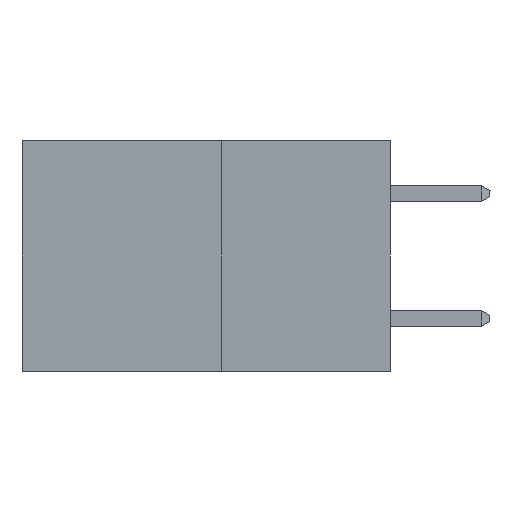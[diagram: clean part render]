
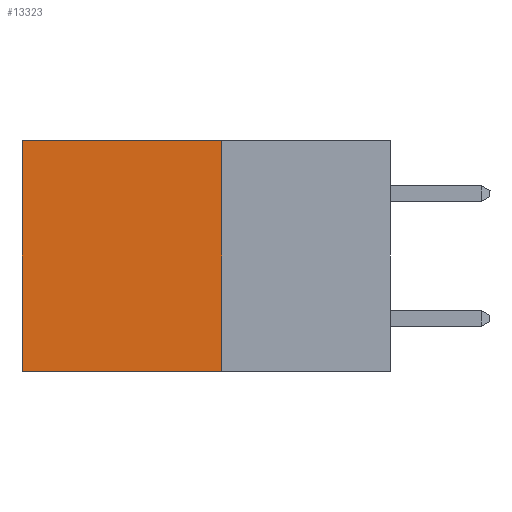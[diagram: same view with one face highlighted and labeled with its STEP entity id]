
A CAD part, left-side view. The second image highlights one B-rep face of the part: STEP entity #13323.
In plain terms, the highlighted planar face has unit normal (-1, 0, 0).
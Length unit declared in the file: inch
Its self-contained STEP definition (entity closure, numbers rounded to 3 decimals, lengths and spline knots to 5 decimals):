
#294 = VECTOR ( 'NONE', #1244, 39.37008 ) ;
#328 = ORIENTED_EDGE ( 'NONE', *, *, #16324, .T. ) ;
#401 = VERTEX_POINT ( 'NONE', #8335 ) ;
#931 = CARTESIAN_POINT ( 'NONE',  ( 0.277, 0.27, -0.37 ) ) ;
#1244 = DIRECTION ( 'NONE',  ( 0., 1., 0. ) ) ;
#3083 = EDGE_CURVE ( 'NONE', #11301, #17555, #4697, .T. ) ;
#3239 = LINE ( 'NONE', #8570, #17644 ) ;
#4622 = AXIS2_PLACEMENT_3D ( 'NONE', #8255, #7303, #7151 ) ;
#4697 = LINE ( 'NONE', #17590, #294 ) ;
#5275 = CARTESIAN_POINT ( 'NONE',  ( 0.277, 0.27, -0.37 ) ) ;
#5292 = DIRECTION ( 'NONE',  ( 0., 0., -1. ) ) ;
#5429 = VECTOR ( 'NONE', #5292, 39.37008 ) ;
#7151 = DIRECTION ( 'NONE',  ( 0., 0., -1. ) ) ;
#7303 = DIRECTION ( 'NONE',  ( 1., 0., 0. ) ) ;
#8029 = CARTESIAN_POINT ( 'NONE',  ( 0.277, 0.27, 0. ) ) ;
#8246 = DIRECTION ( 'NONE',  ( 0., 0., -1. ) ) ;
#8255 = CARTESIAN_POINT ( 'NONE',  ( 0.277, 0.27, -0.37 ) ) ;
#8335 = CARTESIAN_POINT ( 'NONE',  ( 0.277, 0.59, 0. ) ) ;
#8381 = PLANE ( 'NONE',  #4622 ) ;
#8412 = VERTEX_POINT ( 'NONE', #8029 ) ;
#8570 = CARTESIAN_POINT ( 'NONE',  ( 0.277, 0.27, 0. ) ) ;
#8721 = DIRECTION ( 'NONE',  ( 0., 1., 0. ) ) ;
#9347 = ORIENTED_EDGE ( 'NONE', *, *, #10571, .F. ) ;
#9665 = CARTESIAN_POINT ( 'NONE',  ( 0.277, 0.59, -0.37 ) ) ;
#10368 = FACE_OUTER_BOUND ( 'NONE', #12170, .T. ) ;
#10571 = EDGE_CURVE ( 'NONE', #8412, #11301, #16912, .T. ) ;
#11217 = ORIENTED_EDGE ( 'NONE', *, *, #3083, .F. ) ;
#11301 = VERTEX_POINT ( 'NONE', #931 ) ;
#11647 = VECTOR ( 'NONE', #8246, 39.37008 ) ;
#11881 = ORIENTED_EDGE ( 'NONE', *, *, #13999, .T. ) ;
#12170 = EDGE_LOOP ( 'NONE', ( #328, #11217, #9347, #11881 ) ) ;
#13323 = ADVANCED_FACE ( 'NONE', ( #10368 ), #8381, .F. ) ;
#13999 = EDGE_CURVE ( 'NONE', #8412, #401, #3239, .T. ) ;
#14040 = CARTESIAN_POINT ( 'NONE',  ( 0.277, 0.59, -0.37 ) ) ;
#14981 = LINE ( 'NONE', #14040, #11647 ) ;
#16324 = EDGE_CURVE ( 'NONE', #401, #17555, #14981, .T. ) ;
#16912 = LINE ( 'NONE', #5275, #5429 ) ;
#17555 = VERTEX_POINT ( 'NONE', #9665 ) ;
#17590 = CARTESIAN_POINT ( 'NONE',  ( 0.277, 0.27, -0.37 ) ) ;
#17644 = VECTOR ( 'NONE', #8721, 39.37008 ) ;
